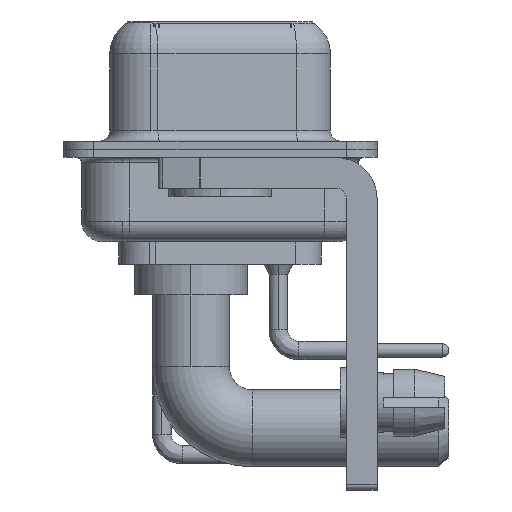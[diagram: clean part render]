
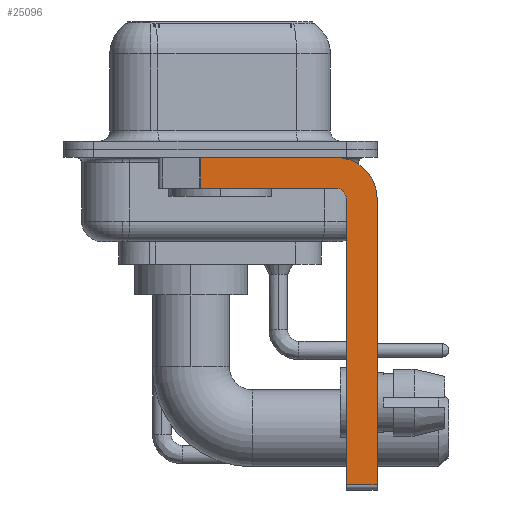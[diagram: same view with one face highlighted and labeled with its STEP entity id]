
A CAD part, left-side view. The second image highlights one B-rep face of the part: STEP entity #25096.
In plain terms, the highlighted planar face has unit normal (-1, 0, 0).
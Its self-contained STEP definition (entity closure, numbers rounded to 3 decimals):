
#417 = CARTESIAN_POINT ( 'NONE',  ( -2.9, 0.978, -1.9 ) ) ;
#585 = CARTESIAN_POINT ( 'NONE',  ( -2.9, -6.15, -16.6 ) ) ;
#754 = CIRCLE ( 'NONE', #18160, 0.5 ) ;
#956 = CARTESIAN_POINT ( 'NONE',  ( -2.9, -6.15, -2.4 ) ) ;
#1057 = LINE ( 'NONE', #585, #30278 ) ;
#2242 = ORIENTED_EDGE ( 'NONE', *, *, #14281, .F. ) ;
#3246 = VERTEX_POINT ( 'NONE', #23469 ) ;
#3388 = CARTESIAN_POINT ( 'NONE',  ( -2.9, -7.65, -2.4 ) ) ;
#3460 = DIRECTION ( 'NONE',  ( 0., 0., 1. ) ) ;
#3494 = CARTESIAN_POINT ( 'NONE',  ( -2.9, -7.65, -2.4 ) ) ;
#4597 = ORIENTED_EDGE ( 'NONE', *, *, #13311, .T. ) ;
#4635 = VERTEX_POINT ( 'NONE', #956 ) ;
#6358 = ORIENTED_EDGE ( 'NONE', *, *, #22395, .F. ) ;
#6778 = DIRECTION ( 'NONE',  ( 0., 0., -1. ) ) ;
#6824 = PLANE ( 'NONE',  #19508 ) ;
#7835 = EDGE_CURVE ( 'NONE', #4635, #23092, #754, .T. ) ;
#8309 = CARTESIAN_POINT ( 'NONE',  ( -2.9, -5.65, -16.35 ) ) ;
#8502 = DIRECTION ( 'NONE',  ( 0., 0., 1. ) ) ;
#8993 = VECTOR ( 'NONE', #25610, 1000. ) ;
#9904 = VECTOR ( 'NONE', #16227, 1000. ) ;
#11004 = FACE_OUTER_BOUND ( 'NONE', #14950, .T. ) ;
#11893 = CARTESIAN_POINT ( 'NONE',  ( -2.9, -5.65, -1.9 ) ) ;
#12457 = DIRECTION ( 'NONE',  ( 0., 0., -1. ) ) ;
#13311 = EDGE_CURVE ( 'NONE', #29886, #17818, #21927, .T. ) ;
#13483 = CARTESIAN_POINT ( 'NONE',  ( -2.9, -5.65, -2.4 ) ) ;
#13549 = VECTOR ( 'NONE', #30447, 1000. ) ;
#13644 = DIRECTION ( 'NONE',  ( -1., 0., 0. ) ) ;
#14000 = CARTESIAN_POINT ( 'NONE',  ( -2.9, -5.65, -2.4 ) ) ;
#14281 = EDGE_CURVE ( 'NONE', #23092, #17818, #26006, .T. ) ;
#14950 = EDGE_LOOP ( 'NONE', ( #22128, #4597, #2242, #30906, #22899, #16017, #15084, #6358 ) ) ;
#15084 = ORIENTED_EDGE ( 'NONE', *, *, #30197, .F. ) ;
#16017 = ORIENTED_EDGE ( 'NONE', *, *, #21706, .T. ) ;
#16227 = DIRECTION ( 'NONE',  ( 0., 1., 0. ) ) ;
#17462 = LINE ( 'NONE', #8309, #26556 ) ;
#17702 = VERTEX_POINT ( 'NONE', #21688 ) ;
#17818 = VERTEX_POINT ( 'NONE', #22316 ) ;
#17827 = EDGE_CURVE ( 'NONE', #29886, #3246, #24709, .T. ) ;
#18160 = AXIS2_PLACEMENT_3D ( 'NONE', #13483, #13644, #8502 ) ;
#19330 = CARTESIAN_POINT ( 'NONE',  ( -2.9, -7.65, -16.35 ) ) ;
#19508 = AXIS2_PLACEMENT_3D ( 'NONE', #28793, #26072, #30580 ) ;
#20233 = CARTESIAN_POINT ( 'NONE',  ( -2.9, 3., -0.4 ) ) ;
#20463 = CIRCLE ( 'NONE', #22522, 2. ) ;
#21688 = CARTESIAN_POINT ( 'NONE',  ( -2.9, -6.15, -16.35 ) ) ;
#21706 = EDGE_CURVE ( 'NONE', #17702, #23884, #17462, .T. ) ;
#21901 = CARTESIAN_POINT ( 'NONE',  ( -2.9, 0.978, -0.4 ) ) ;
#21927 = LINE ( 'NONE', #417, #23517 ) ;
#22128 = ORIENTED_EDGE ( 'NONE', *, *, #17827, .F. ) ;
#22316 = CARTESIAN_POINT ( 'NONE',  ( -2.9, 0.978, -1.9 ) ) ;
#22395 = EDGE_CURVE ( 'NONE', #3246, #31670, #20463, .T. ) ;
#22522 = AXIS2_PLACEMENT_3D ( 'NONE', #14000, #23768, #6778 ) ;
#22752 = DIRECTION ( 'NONE',  ( 0., -1., 0. ) ) ;
#22899 = ORIENTED_EDGE ( 'NONE', *, *, #23511, .F. ) ;
#23092 = VERTEX_POINT ( 'NONE', #30301 ) ;
#23469 = CARTESIAN_POINT ( 'NONE',  ( -2.9, -5.65, -0.4 ) ) ;
#23511 = EDGE_CURVE ( 'NONE', #17702, #4635, #1057, .T. ) ;
#23517 = VECTOR ( 'NONE', #12457, 1000. ) ;
#23768 = DIRECTION ( 'NONE',  ( 1., 0., 0. ) ) ;
#23884 = VERTEX_POINT ( 'NONE', #19330 ) ;
#24709 = LINE ( 'NONE', #20233, #8993 ) ;
#25096 = ADVANCED_FACE ( 'NONE', ( #11004 ), #6824, .F. ) ;
#25610 = DIRECTION ( 'NONE',  ( 0., -1., 0. ) ) ;
#25776 = LINE ( 'NONE', #3494, #13549 ) ;
#26006 = LINE ( 'NONE', #11893, #9904 ) ;
#26072 = DIRECTION ( 'NONE',  ( 1., 0., 0. ) ) ;
#26556 = VECTOR ( 'NONE', #22752, 1000. ) ;
#28793 = CARTESIAN_POINT ( 'NONE',  ( -2.9, -5.65, -2.4 ) ) ;
#29886 = VERTEX_POINT ( 'NONE', #21901 ) ;
#30197 = EDGE_CURVE ( 'NONE', #31670, #23884, #25776, .T. ) ;
#30278 = VECTOR ( 'NONE', #3460, 1000. ) ;
#30301 = CARTESIAN_POINT ( 'NONE',  ( -2.9, -5.65, -1.9 ) ) ;
#30447 = DIRECTION ( 'NONE',  ( 0., 0., -1. ) ) ;
#30580 = DIRECTION ( 'NONE',  ( 0., 0., -1. ) ) ;
#30906 = ORIENTED_EDGE ( 'NONE', *, *, #7835, .F. ) ;
#31670 = VERTEX_POINT ( 'NONE', #3388 ) ;
